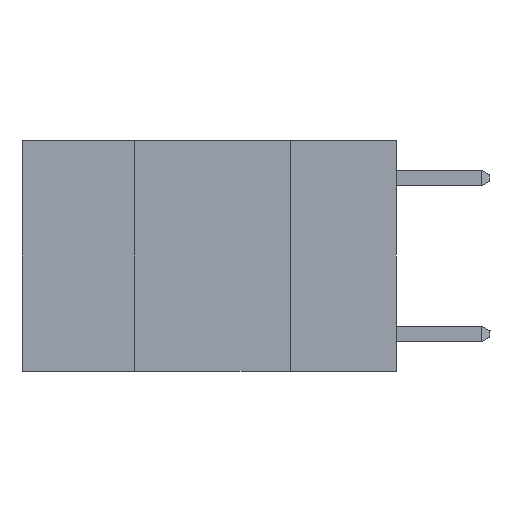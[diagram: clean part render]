
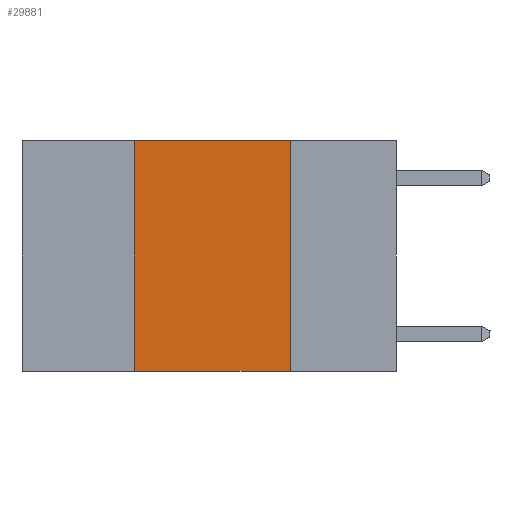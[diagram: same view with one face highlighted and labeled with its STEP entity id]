
A CAD part, left-side view. The second image highlights one B-rep face of the part: STEP entity #29881.
In plain terms, the highlighted planar face has unit normal (-1, 0, 0).
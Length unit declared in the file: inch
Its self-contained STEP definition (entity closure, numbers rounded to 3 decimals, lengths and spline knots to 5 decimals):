
#627 = VECTOR ( 'NONE', #26809, 39.37008 ) ;
#1168 = CARTESIAN_POINT ( 'NONE',  ( 0., 0.6, 0. ) ) ;
#1423 = LINE ( 'NONE', #12764, #627 ) ;
#2427 = VECTOR ( 'NONE', #17145, 39.37008 ) ;
#3751 = CARTESIAN_POINT ( 'NONE',  ( 0., 0.17, 0. ) ) ;
#5608 = CARTESIAN_POINT ( 'NONE',  ( 0., 0.17, 0. ) ) ;
#5984 = LINE ( 'NONE', #1168, #18797 ) ;
#6234 = DIRECTION ( 'NONE',  ( 0., 0., -1. ) ) ;
#6391 = VERTEX_POINT ( 'NONE', #28759 ) ;
#6835 = VERTEX_POINT ( 'NONE', #19523 ) ;
#7749 = ORIENTED_EDGE ( 'NONE', *, *, #18148, .T. ) ;
#8003 = CARTESIAN_POINT ( 'NONE',  ( 0., 0.6, 0. ) ) ;
#9583 = ORIENTED_EDGE ( 'NONE', *, *, #26257, .F. ) ;
#9749 = EDGE_CURVE ( 'NONE', #6391, #12990, #5984, .T. ) ;
#10397 = DIRECTION ( 'NONE',  ( 0., 0., -1. ) ) ;
#11250 = FACE_OUTER_BOUND ( 'NONE', #18515, .T. ) ;
#11797 = VERTEX_POINT ( 'NONE', #30075 ) ;
#12304 = LINE ( 'NONE', #3751, #17923 ) ;
#12764 = CARTESIAN_POINT ( 'NONE',  ( 0., 0.6, -0.37 ) ) ;
#12990 = VERTEX_POINT ( 'NONE', #5608 ) ;
#14739 = CARTESIAN_POINT ( 'NONE',  ( 0., 0.42, 0. ) ) ;
#17145 = DIRECTION ( 'NONE',  ( 0., 0., 1. ) ) ;
#17546 = PLANE ( 'NONE',  #21391 ) ;
#17923 = VECTOR ( 'NONE', #6234, 39.37008 ) ;
#18136 = DIRECTION ( 'NONE',  ( 0., -1., 0. ) ) ;
#18148 = EDGE_CURVE ( 'NONE', #6835, #11797, #1423, .T. ) ;
#18515 = EDGE_LOOP ( 'NONE', ( #29030, #25787, #9583, #7749 ) ) ;
#18797 = VECTOR ( 'NONE', #18136, 39.37008 ) ;
#19523 = CARTESIAN_POINT ( 'NONE',  ( 0., 0.42, -0.37 ) ) ;
#21391 = AXIS2_PLACEMENT_3D ( 'NONE', #8003, #24569, #10397 ) ;
#21609 = LINE ( 'NONE', #14739, #2427 ) ;
#24569 = DIRECTION ( 'NONE',  ( 1., 0., 0. ) ) ;
#25787 = ORIENTED_EDGE ( 'NONE', *, *, #9749, .F. ) ;
#26257 = EDGE_CURVE ( 'NONE', #6835, #6391, #21609, .T. ) ;
#26809 = DIRECTION ( 'NONE',  ( 0., -1., 0. ) ) ;
#27239 = EDGE_CURVE ( 'NONE', #12990, #11797, #12304, .T. ) ;
#28759 = CARTESIAN_POINT ( 'NONE',  ( 0., 0.42, 0. ) ) ;
#29030 = ORIENTED_EDGE ( 'NONE', *, *, #27239, .F. ) ;
#29881 = ADVANCED_FACE ( 'NONE', ( #11250 ), #17546, .F. ) ;
#30075 = CARTESIAN_POINT ( 'NONE',  ( 0., 0.17, -0.37 ) ) ;
